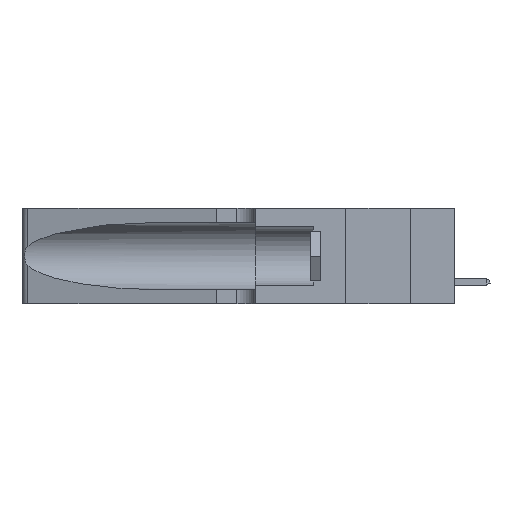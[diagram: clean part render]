
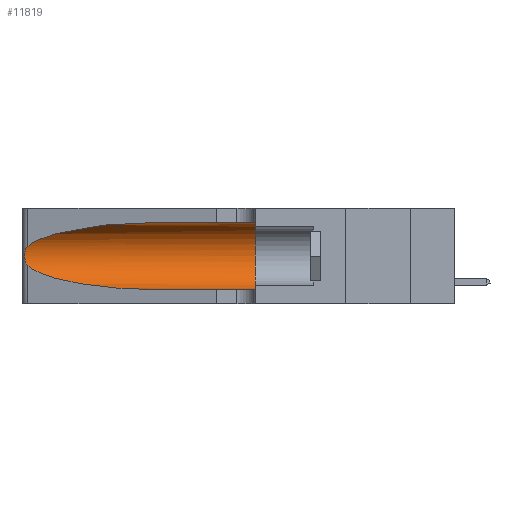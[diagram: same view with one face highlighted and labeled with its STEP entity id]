
A CAD part, left-side view. The second image highlights one B-rep face of the part: STEP entity #11819.
In plain terms, the highlighted cylindrical face has radius 3.308 mm (diameter 6.617 mm), a partial arc.
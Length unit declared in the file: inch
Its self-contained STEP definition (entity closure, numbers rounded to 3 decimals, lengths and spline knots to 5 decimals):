
#120 = ORIENTED_EDGE ( 'NONE', *, *, #14756, .F. ) ;
#609 = ORIENTED_EDGE ( 'NONE', *, *, #4670, .T. ) ;
#1015 = CARTESIAN_POINT ( 'NONE',  ( 0.25487, 1.22718, 0.22369 ) ) ;
#1310 = B_SPLINE_CURVE_WITH_KNOTS ( 'NONE', 3,
 ( #3576, #14909, #16557, #18183, #13284, #3710, #11452, #1790, #8333, #16334, #19587, #1921, #3430, #5076 ),
 .UNSPECIFIED., .F., .F.,
 ( 4, 2, 2, 2, 2, 2, 4 ),
 ( 0., 0.00027, 0.00053, 0.00107, 0.0016, 0.00187, 0.00214 ),
 .UNSPECIFIED. ) ;
#1523 = CARTESIAN_POINT ( 'NONE',  ( 0.2373, 1.15595, 0.08982 ) ) ;
#1602 = CARTESIAN_POINT ( 'NONE',  ( 0.1305, 0.72297, 0.05475 ) ) ;
#1790 = CARTESIAN_POINT ( 'NONE',  ( 0.26075, 1.23896, 0.178 ) ) ;
#1921 = CARTESIAN_POINT ( 'NONE',  ( 0.25639, 1.23186, 0.15144 ) ) ;
#2866 = CARTESIAN_POINT ( 'NONE',  ( 0.1305, 0.72297, 0.31525 ) ) ;
#3430 = CARTESIAN_POINT ( 'NONE',  ( 0.25555, 1.22993, 0.14849 ) ) ;
#3576 = CARTESIAN_POINT ( 'NONE',  ( 0.25487, 1.22718, 0.22369 ) ) ;
#3710 = CARTESIAN_POINT ( 'NONE',  ( 0.26018, 1.23835, 0.19895 ) ) ;
#3735 = CARTESIAN_POINT ( 'NONE',  ( 0.1305, 1.61858, 0.05475 ) ) ;
#4606 = CARTESIAN_POINT ( 'NONE',  ( 0.18966, 0.96281, 0.05475 ) ) ;
#4670 = EDGE_CURVE ( 'NONE', #16728, #8068, #18540, .T. ) ;
#4969 = EDGE_CURVE ( 'NONE', #16787, #16658, #18630, .T. ) ;
#5076 = CARTESIAN_POINT ( 'NONE',  ( 0.25487, 1.22718, 0.14631 ) ) ;
#5299 = CARTESIAN_POINT ( 'NONE',  ( 0.25487, 1.22718, 0.22369 ) ) ;
#5936 = CARTESIAN_POINT ( 'NONE',  ( 0.1305, 0.72297, 0.31525 ) ) ;
#6196 = ORIENTED_EDGE ( 'NONE', *, *, #10682, .T. ) ;
#6704 = LINE ( 'NONE', #3735, #10463 ) ;
#6964 = DIRECTION ( 'NONE',  ( 0., -1., 0. ) ) ;
#7290 = CARTESIAN_POINT ( 'NONE',  ( 0.1305, 0.72297, 0.05475 ) ) ;
#8068 = VERTEX_POINT ( 'NONE', #7290 ) ;
#8333 = CARTESIAN_POINT ( 'NONE',  ( 0.26017, 1.23833, 0.17102 ) ) ;
#8553 = DIRECTION ( 'NONE',  ( 0., 0., -1. ) ) ;
#9892 = AXIS2_PLACEMENT_3D ( 'NONE', #11443, #18173, #18589 ) ;
#10463 = VECTOR ( 'NONE', #11966, 39.37008 ) ;
#10682 = EDGE_CURVE ( 'NONE', #8068, #16658, #6704, .T. ) ;
#11413 = DIRECTION ( 'NONE',  ( 0., -1., 0. ) ) ;
#11419 = EDGE_CURVE ( 'NONE', #14432, #16728, #1310, .T. ) ;
#11443 = CARTESIAN_POINT ( 'NONE',  ( 0.1305, 0.35, 0.185 ) ) ;
#11452 = CARTESIAN_POINT ( 'NONE',  ( 0.26075, 1.23896, 0.19203 ) ) ;
#11520 = CARTESIAN_POINT ( 'NONE',  ( 0.25487, 1.22718, 0.14631 ) ) ;
#11819 = ADVANCED_FACE ( 'NONE', ( #17350 ), #13788, .F. ) ;
#11966 = DIRECTION ( 'NONE',  ( 0., -1., 0. ) ) ;
#12539 = EDGE_CURVE ( 'NONE', #16416, #14432, #13856, .T. ) ;
#12594 = CARTESIAN_POINT ( 'NONE',  ( 0.2373, 1.15595, 0.28018 ) ) ;
#13080 = CARTESIAN_POINT ( 'NONE',  ( 0.1305, 0.35, 0.05475 ) ) ;
#13284 = CARTESIAN_POINT ( 'NONE',  ( 0.25854, 1.2359, 0.20912 ) ) ;
#13420 = ORIENTED_EDGE ( 'NONE', *, *, #11419, .T. ) ;
#13788 = CYLINDRICAL_SURFACE ( 'NONE', #14677, 0.13025 ) ;
#13856 =( BOUNDED_CURVE ( )  B_SPLINE_CURVE ( 3, ( #5936, #17347, #12594, #1015 ),
 .UNSPECIFIED., .F., .T. ) 
 B_SPLINE_CURVE_WITH_KNOTS ( ( 4, 4 ),
 ( 1.5708, 2.84003 ),
 .UNSPECIFIED. ) 
 CURVE ( )  GEOMETRIC_REPRESENTATION_ITEM ( )  RATIONAL_B_SPLINE_CURVE ( ( 1., 0.87, 0.87, 1. ) ) 
 REPRESENTATION_ITEM ( '' )  );
#14432 = VERTEX_POINT ( 'NONE', #5299 ) ;
#14677 = AXIS2_PLACEMENT_3D ( 'NONE', #16705, #6964, #8553 ) ;
#14756 = EDGE_CURVE ( 'NONE', #16416, #16787, #17712, .T. ) ;
#14909 = CARTESIAN_POINT ( 'NONE',  ( 0.25555, 1.22994, 0.2215 ) ) ;
#15256 = CARTESIAN_POINT ( 'NONE',  ( 0.1305, 0.35, 0.31525 ) ) ;
#15876 = CARTESIAN_POINT ( 'NONE',  ( 0.1305, 1.61858, 0.31525 ) ) ;
#15943 = CARTESIAN_POINT ( 'NONE',  ( 0.25487, 1.22718, 0.14631 ) ) ;
#16112 = EDGE_LOOP ( 'NONE', ( #19244, #13420, #609, #6196, #20701, #120 ) ) ;
#16334 = CARTESIAN_POINT ( 'NONE',  ( 0.25856, 1.23593, 0.16098 ) ) ;
#16416 = VERTEX_POINT ( 'NONE', #2866 ) ;
#16557 = CARTESIAN_POINT ( 'NONE',  ( 0.25639, 1.23184, 0.21858 ) ) ;
#16658 = VERTEX_POINT ( 'NONE', #13080 ) ;
#16705 = CARTESIAN_POINT ( 'NONE',  ( 0.1305, 1.61858, 0.185 ) ) ;
#16728 = VERTEX_POINT ( 'NONE', #11520 ) ;
#16787 = VERTEX_POINT ( 'NONE', #15256 ) ;
#17347 = CARTESIAN_POINT ( 'NONE',  ( 0.18966, 0.96281, 0.31525 ) ) ;
#17350 = FACE_OUTER_BOUND ( 'NONE', #16112, .T. ) ;
#17712 = LINE ( 'NONE', #15876, #19734 ) ;
#18173 = DIRECTION ( 'NONE',  ( 0., 1., 0. ) ) ;
#18183 = CARTESIAN_POINT ( 'NONE',  ( 0.25787, 1.23484, 0.2124 ) ) ;
#18540 =( BOUNDED_CURVE ( )  B_SPLINE_CURVE ( 3, ( #15943, #1523, #4606, #1602 ),
 .UNSPECIFIED., .F., .T. ) 
 B_SPLINE_CURVE_WITH_KNOTS ( ( 4, 4 ),
 ( 3.44316, 4.71239 ),
 .UNSPECIFIED. ) 
 CURVE ( )  GEOMETRIC_REPRESENTATION_ITEM ( )  RATIONAL_B_SPLINE_CURVE ( ( 1., 0.87, 0.87, 1. ) ) 
 REPRESENTATION_ITEM ( '' )  );
#18589 = DIRECTION ( 'NONE',  ( 0., 0., 1. ) ) ;
#18630 = CIRCLE ( 'NONE', #9892, 0.13025 ) ;
#19244 = ORIENTED_EDGE ( 'NONE', *, *, #12539, .T. ) ;
#19587 = CARTESIAN_POINT ( 'NONE',  ( 0.25789, 1.23486, 0.15765 ) ) ;
#19734 = VECTOR ( 'NONE', #11413, 39.37008 ) ;
#20701 = ORIENTED_EDGE ( 'NONE', *, *, #4969, .F. ) ;
